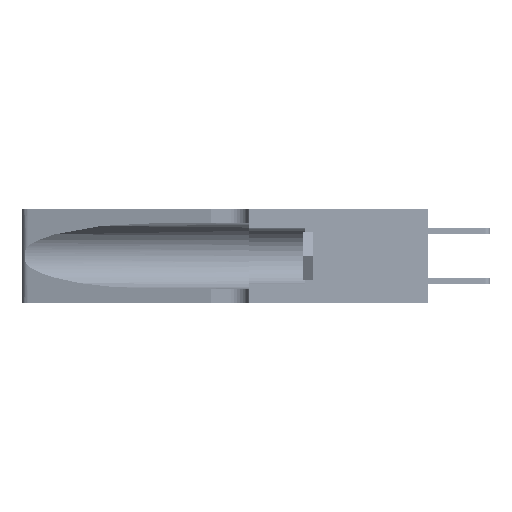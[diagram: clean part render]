
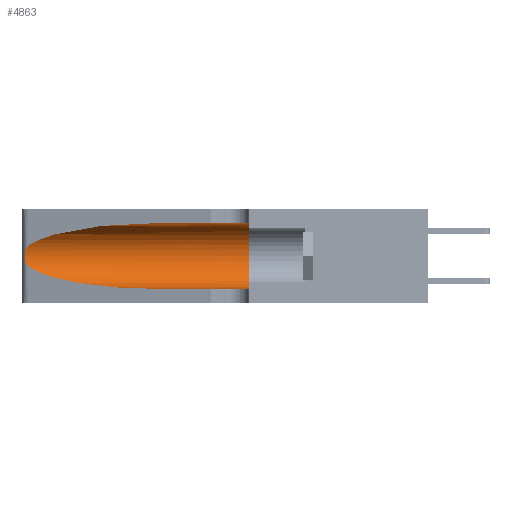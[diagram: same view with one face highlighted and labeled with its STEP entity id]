
A CAD part, left-side view. The second image highlights one B-rep face of the part: STEP entity #4863.
In plain terms, the highlighted cylindrical face has radius 3.308 mm (diameter 6.617 mm), a partial arc.
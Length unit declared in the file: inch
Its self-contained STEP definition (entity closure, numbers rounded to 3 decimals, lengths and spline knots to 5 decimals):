
#537 = EDGE_CURVE ( 'NONE', #34219, #29920, #18755, .T. ) ;
#1567 = FACE_OUTER_BOUND ( 'NONE', #22189, .T. ) ;
#1643 = CARTESIAN_POINT ( 'NONE',  ( 0.1305, 0.35, 0.31525 ) ) ;
#4863 = ADVANCED_FACE ( 'NONE', ( #1567 ), #24262, .F. ) ;
#6181 = CARTESIAN_POINT ( 'NONE',  ( 0.25487, 1.22718, 0.14631 ) ) ;
#7221 = CARTESIAN_POINT ( 'NONE',  ( 0.25856, 1.23593, 0.16098 ) ) ;
#7490 = ORIENTED_EDGE ( 'NONE', *, *, #20774, .F. ) ;
#7749 = VECTOR ( 'NONE', #40129, 39.37008 ) ;
#8528 = CARTESIAN_POINT ( 'NONE',  ( 0.18966, 0.96281, 0.31525 ) ) ;
#8541 = ORIENTED_EDGE ( 'NONE', *, *, #13713, .T. ) ;
#9128 = VECTOR ( 'NONE', #17804, 39.37008 ) ;
#10933 = CARTESIAN_POINT ( 'NONE',  ( 0.25487, 1.22718, 0.14631 ) ) ;
#10997 = ORIENTED_EDGE ( 'NONE', *, *, #19731, .T. ) ;
#11949 = CARTESIAN_POINT ( 'NONE',  ( 0.1305, 0.35, 0.05475 ) ) ;
#12043 = CARTESIAN_POINT ( 'NONE',  ( 0.25487, 1.22718, 0.22369 ) ) ;
#12044 = CARTESIAN_POINT ( 'NONE',  ( 0.1305, 0.35, 0.185 ) ) ;
#12571 = VERTEX_POINT ( 'NONE', #13247 ) ;
#13197 = AXIS2_PLACEMENT_3D ( 'NONE', #12044, #15838, #19773 ) ;
#13247 = CARTESIAN_POINT ( 'NONE',  ( 0.25487, 1.22718, 0.22369 ) ) ;
#13396 = VERTEX_POINT ( 'NONE', #10933 ) ;
#13713 = EDGE_CURVE ( 'NONE', #25447, #12571, #25931, .T. ) ;
#14191 = CARTESIAN_POINT ( 'NONE',  ( 0.1305, 1.61858, 0.05475 ) ) ;
#14225 = CARTESIAN_POINT ( 'NONE',  ( 0.26075, 1.23896, 0.178 ) ) ;
#15838 = DIRECTION ( 'NONE',  ( 0., 1., 0. ) ) ;
#16826 = DIRECTION ( 'NONE',  ( 0., 0., -1. ) ) ;
#17380 = CARTESIAN_POINT ( 'NONE',  ( 0.25639, 1.23184, 0.21858 ) ) ;
#17690 = CARTESIAN_POINT ( 'NONE',  ( 0.26017, 1.23833, 0.17102 ) ) ;
#17804 = DIRECTION ( 'NONE',  ( 0., -1., 0. ) ) ;
#18755 = LINE ( 'NONE', #14191, #9128 ) ;
#19048 = DIRECTION ( 'NONE',  ( 0., -1., 0. ) ) ;
#19731 = EDGE_CURVE ( 'NONE', #13396, #34219, #25350, .T. ) ;
#19773 = DIRECTION ( 'NONE',  ( 0., 0., 1. ) ) ;
#20774 = EDGE_CURVE ( 'NONE', #25447, #24006, #34358, .T. ) ;
#21148 = CARTESIAN_POINT ( 'NONE',  ( 0.25639, 1.23186, 0.15144 ) ) ;
#21459 = CARTESIAN_POINT ( 'NONE',  ( 0.25789, 1.23486, 0.15765 ) ) ;
#22064 = CARTESIAN_POINT ( 'NONE',  ( 0.1305, 1.61858, 0.185 ) ) ;
#22189 = EDGE_LOOP ( 'NONE', ( #8541, #38349, #10997, #32667, #25312, #7490 ) ) ;
#23913 = CARTESIAN_POINT ( 'NONE',  ( 0.1305, 0.72297, 0.05475 ) ) ;
#24006 = VERTEX_POINT ( 'NONE', #1643 ) ;
#24262 = CYLINDRICAL_SURFACE ( 'NONE', #32703, 0.13025 ) ;
#25312 = ORIENTED_EDGE ( 'NONE', *, *, #34113, .F. ) ;
#25350 =( BOUNDED_CURVE ( )  B_SPLINE_CURVE ( 3, ( #6181, #41948, #34813, #23913 ),
 .UNSPECIFIED., .F., .F. ) 
 B_SPLINE_CURVE_WITH_KNOTS ( ( 4, 4 ),
 ( 3.44316, 4.71239 ),
 .UNSPECIFIED. ) 
 CURVE ( )  GEOMETRIC_REPRESENTATION_ITEM ( )  RATIONAL_B_SPLINE_CURVE ( ( 1., 0.87, 0.87, 1. ) ) 
 REPRESENTATION_ITEM ( '' )  );
#25447 = VERTEX_POINT ( 'NONE', #45220 ) ;
#25911 = CARTESIAN_POINT ( 'NONE',  ( 0.1305, 1.61858, 0.31525 ) ) ;
#25931 =( BOUNDED_CURVE ( )  B_SPLINE_CURVE ( 3, ( #30244, #8528, #26943, #12043 ),
 .UNSPECIFIED., .F., .T. ) 
 B_SPLINE_CURVE_WITH_KNOTS ( ( 4, 4 ),
 ( 1.5708, 2.84003 ),
 .UNSPECIFIED. ) 
 CURVE ( )  GEOMETRIC_REPRESENTATION_ITEM ( )  RATIONAL_B_SPLINE_CURVE ( ( 1., 0.87, 0.87, 1. ) ) 
 REPRESENTATION_ITEM ( '' )  );
#26943 = CARTESIAN_POINT ( 'NONE',  ( 0.2373, 1.15595, 0.28018 ) ) ;
#28814 = B_SPLINE_CURVE_WITH_KNOTS ( 'NONE', 3,
 ( #39216, #46663, #17380, #39676, #39371, #31932, #35882, #14225, #17690, #7221, #21459, #21148, #43007, #46821 ),
 .UNSPECIFIED., .F., .F.,
 ( 4, 2, 2, 2, 2, 2, 4 ),
 ( 0., 0.00027, 0.00053, 0.00107, 0.0016, 0.00187, 0.00214 ),
 .UNSPECIFIED. ) ;
#29920 = VERTEX_POINT ( 'NONE', #11949 ) ;
#30244 = CARTESIAN_POINT ( 'NONE',  ( 0.1305, 0.72297, 0.31525 ) ) ;
#31932 = CARTESIAN_POINT ( 'NONE',  ( 0.26018, 1.23835, 0.19895 ) ) ;
#32667 = ORIENTED_EDGE ( 'NONE', *, *, #537, .T. ) ;
#32703 = AXIS2_PLACEMENT_3D ( 'NONE', #22064, #19048, #16826 ) ;
#34113 = EDGE_CURVE ( 'NONE', #24006, #29920, #36510, .T. ) ;
#34219 = VERTEX_POINT ( 'NONE', #45261 ) ;
#34358 = LINE ( 'NONE', #25911, #7749 ) ;
#34813 = CARTESIAN_POINT ( 'NONE',  ( 0.18966, 0.96281, 0.05475 ) ) ;
#35882 = CARTESIAN_POINT ( 'NONE',  ( 0.26075, 1.23896, 0.19203 ) ) ;
#36510 = CIRCLE ( 'NONE', #13197, 0.13025 ) ;
#38349 = ORIENTED_EDGE ( 'NONE', *, *, #44351, .T. ) ;
#39216 = CARTESIAN_POINT ( 'NONE',  ( 0.25487, 1.22718, 0.22369 ) ) ;
#39371 = CARTESIAN_POINT ( 'NONE',  ( 0.25854, 1.2359, 0.20912 ) ) ;
#39676 = CARTESIAN_POINT ( 'NONE',  ( 0.25787, 1.23484, 0.2124 ) ) ;
#40129 = DIRECTION ( 'NONE',  ( 0., -1., 0. ) ) ;
#41948 = CARTESIAN_POINT ( 'NONE',  ( 0.2373, 1.15595, 0.08982 ) ) ;
#43007 = CARTESIAN_POINT ( 'NONE',  ( 0.25555, 1.22993, 0.14849 ) ) ;
#44351 = EDGE_CURVE ( 'NONE', #12571, #13396, #28814, .T. ) ;
#45220 = CARTESIAN_POINT ( 'NONE',  ( 0.1305, 0.72297, 0.31525 ) ) ;
#45261 = CARTESIAN_POINT ( 'NONE',  ( 0.1305, 0.72297, 0.05475 ) ) ;
#46663 = CARTESIAN_POINT ( 'NONE',  ( 0.25555, 1.22994, 0.2215 ) ) ;
#46821 = CARTESIAN_POINT ( 'NONE',  ( 0.25487, 1.22718, 0.14631 ) ) ;
